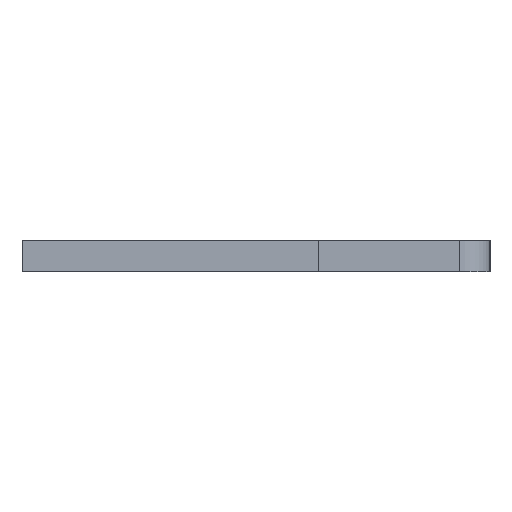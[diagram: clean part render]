
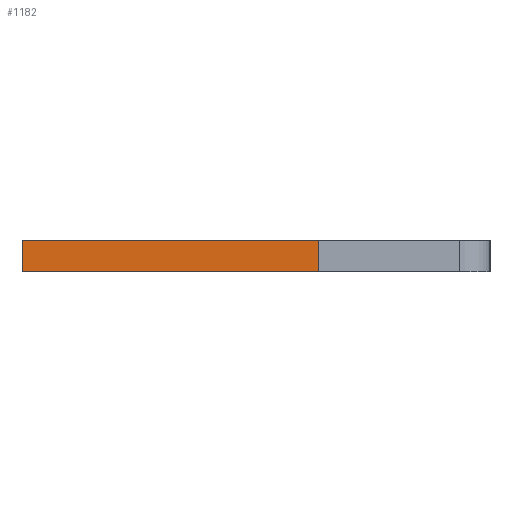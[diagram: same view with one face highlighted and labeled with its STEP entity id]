
A CAD part, left-side view. The second image highlights one B-rep face of the part: STEP entity #1182.
In plain terms, the highlighted face is planar.
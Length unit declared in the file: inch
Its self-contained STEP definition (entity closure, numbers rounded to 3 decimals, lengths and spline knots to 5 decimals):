
#3 = CARTESIAN_POINT ( 'NONE',  ( 0.01, 0.15, -0.04 ) ) ;
#108 = VERTEX_POINT ( 'NONE', #1959 ) ;
#142 = LINE ( 'NONE', #774, #1380 ) ;
#145 = ORIENTED_EDGE ( 'NONE', *, *, #1317, .T. ) ;
#212 = VERTEX_POINT ( 'NONE', #2124 ) ;
#232 = DIRECTION ( 'NONE',  ( 0., 0., 1. ) ) ;
#398 = LINE ( 'NONE', #1562, #2514 ) ;
#413 = PLANE ( 'NONE',  #832 ) ;
#514 = LINE ( 'NONE', #1719, #1480 ) ;
#658 = EDGE_CURVE ( 'NONE', #108, #888, #398, .T. ) ;
#774 = CARTESIAN_POINT ( 'NONE',  ( 0.01, 0.15, -0.04 ) ) ;
#832 = AXIS2_PLACEMENT_3D ( 'NONE', #1269, #232, #1882 ) ;
#855 = CARTESIAN_POINT ( 'NONE',  ( -0.01, 0.15, -0.04 ) ) ;
#870 = VERTEX_POINT ( 'NONE', #1403 ) ;
#888 = VERTEX_POINT ( 'NONE', #3 ) ;
#921 = EDGE_CURVE ( 'NONE', #888, #212, #142, .T. ) ;
#959 = DIRECTION ( 'NONE',  ( 0., 1., 0. ) ) ;
#1182 = ADVANCED_FACE ( 'NONE', ( #1321 ), #413, .F. ) ;
#1226 = DIRECTION ( 'NONE',  ( 0., 1., 0. ) ) ;
#1269 = CARTESIAN_POINT ( 'NONE',  ( 0.01, 0.15, -0.04 ) ) ;
#1317 = EDGE_CURVE ( 'NONE', #870, #212, #2269, .T. ) ;
#1321 = FACE_OUTER_BOUND ( 'NONE', #2182, .T. ) ;
#1380 = VECTOR ( 'NONE', #2040, 39.37008 ) ;
#1403 = CARTESIAN_POINT ( 'NONE',  ( -0.01, -0.04, -0.04 ) ) ;
#1480 = VECTOR ( 'NONE', #1535, 39.37008 ) ;
#1535 = DIRECTION ( 'NONE',  ( -1., 0., 0. ) ) ;
#1562 = CARTESIAN_POINT ( 'NONE',  ( 0.01, 0.15, -0.04 ) ) ;
#1566 = VECTOR ( 'NONE', #1226, 39.37008 ) ;
#1596 = ORIENTED_EDGE ( 'NONE', *, *, #658, .F. ) ;
#1719 = CARTESIAN_POINT ( 'NONE',  ( 0.01, -0.04, -0.04 ) ) ;
#1882 = DIRECTION ( 'NONE',  ( 1., 0., 0. ) ) ;
#1926 = ORIENTED_EDGE ( 'NONE', *, *, #2496, .T. ) ;
#1959 = CARTESIAN_POINT ( 'NONE',  ( 0.01, -0.04, -0.04 ) ) ;
#2040 = DIRECTION ( 'NONE',  ( -1., 0., 0. ) ) ;
#2124 = CARTESIAN_POINT ( 'NONE',  ( -0.01, 0.15, -0.04 ) ) ;
#2182 = EDGE_LOOP ( 'NONE', ( #145, #2311, #1596, #1926 ) ) ;
#2269 = LINE ( 'NONE', #855, #1566 ) ;
#2311 = ORIENTED_EDGE ( 'NONE', *, *, #921, .F. ) ;
#2496 = EDGE_CURVE ( 'NONE', #108, #870, #514, .T. ) ;
#2514 = VECTOR ( 'NONE', #959, 39.37008 ) ;
